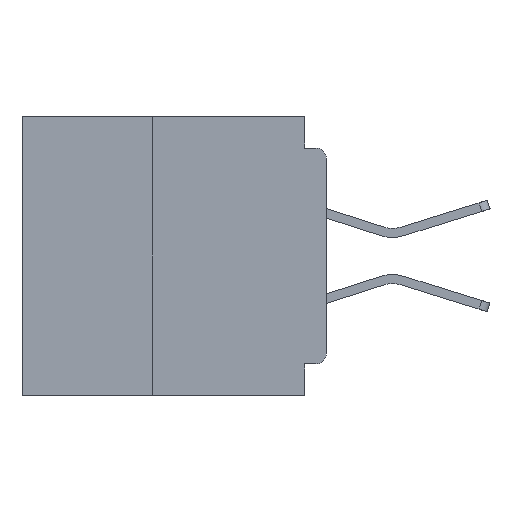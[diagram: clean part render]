
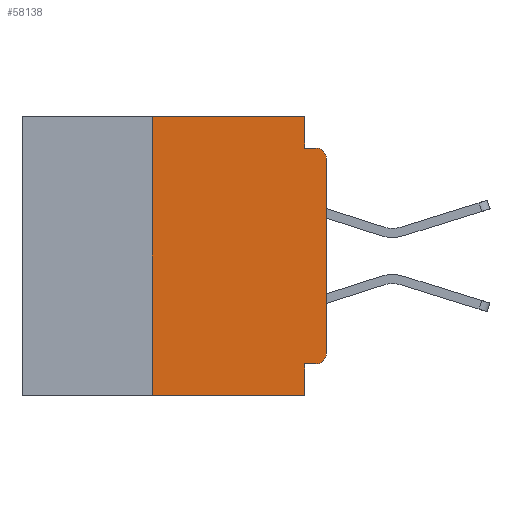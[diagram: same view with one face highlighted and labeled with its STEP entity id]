
A CAD part, left-side view. The second image highlights one B-rep face of the part: STEP entity #58138.
In plain terms, the highlighted planar face has unit normal (-1, 0, 0).
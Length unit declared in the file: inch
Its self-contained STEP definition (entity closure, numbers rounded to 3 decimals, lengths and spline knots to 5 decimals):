
#1489 = CARTESIAN_POINT ( 'NONE',  ( 0., 0., -0.06 ) ) ;
#2275 = CARTESIAN_POINT ( 'NONE',  ( 0., 0.031, 0. ) ) ;
#2731 = ORIENTED_EDGE ( 'NONE', *, *, #26968, .F. ) ;
#3006 = FACE_OUTER_BOUND ( 'NONE', #5489, .T. ) ;
#3171 = CARTESIAN_POINT ( 'NONE',  ( 0., 0.437, -0.4 ) ) ;
#3813 = VERTEX_POINT ( 'NONE', #17978 ) ;
#4957 = DIRECTION ( 'NONE',  ( 0., 0., 1. ) ) ;
#5137 = EDGE_CURVE ( 'NONE', #26062, #48264, #26834, .T. ) ;
#5148 = VECTOR ( 'NONE', #8338, 39.37008 ) ;
#5489 = EDGE_LOOP ( 'NONE', ( #11112, #23788, #39793, #32274, #34479, #48399, #5959, #2731, #17538, #36929 ) ) ;
#5654 = DIRECTION ( 'NONE',  ( 0., -1., 0. ) ) ;
#5959 = ORIENTED_EDGE ( 'NONE', *, *, #33582, .T. ) ;
#6021 = VERTEX_POINT ( 'NONE', #2275 ) ;
#7006 = EDGE_CURVE ( 'NONE', #56599, #48264, #22376, .T. ) ;
#8338 = DIRECTION ( 'NONE',  ( 0., -1., 0. ) ) ;
#9839 = VERTEX_POINT ( 'NONE', #38324 ) ;
#11072 = CARTESIAN_POINT ( 'NONE',  ( 0., 0.015, -0.34 ) ) ;
#11112 = ORIENTED_EDGE ( 'NONE', *, *, #22814, .T. ) ;
#13249 = CARTESIAN_POINT ( 'NONE',  ( 0., 0., -0.34 ) ) ;
#13445 = PLANE ( 'NONE',  #36985 ) ;
#14200 = CARTESIAN_POINT ( 'NONE',  ( 0., 0.015, -0.355 ) ) ;
#14259 = CARTESIAN_POINT ( 'NONE',  ( 0., 0.015, -0.06 ) ) ;
#14499 = LINE ( 'NONE', #41904, #27992 ) ;
#14874 = DIRECTION ( 'NONE',  ( 0., 1., 0. ) ) ;
#15630 = DIRECTION ( 'NONE',  ( 0., 0., -1. ) ) ;
#15674 = VECTOR ( 'NONE', #28658, 39.37008 ) ;
#17348 = CARTESIAN_POINT ( 'NONE',  ( 0., 0.031, -0.355 ) ) ;
#17538 = ORIENTED_EDGE ( 'NONE', *, *, #51040, .F. ) ;
#17776 = EDGE_CURVE ( 'NONE', #9839, #3813, #32644, .T. ) ;
#17978 = CARTESIAN_POINT ( 'NONE',  ( 0., 0.25, 0. ) ) ;
#18858 = DIRECTION ( 'NONE',  ( 0., 0., -1. ) ) ;
#21044 = AXIS2_PLACEMENT_3D ( 'NONE', #11072, #42638, #15630 ) ;
#22376 = LINE ( 'NONE', #41868, #56713 ) ;
#22814 = EDGE_CURVE ( 'NONE', #41666, #26062, #39669, .T. ) ;
#23788 = ORIENTED_EDGE ( 'NONE', *, *, #5137, .T. ) ;
#25948 = VECTOR ( 'NONE', #48443, 39.37008 ) ;
#26062 = VERTEX_POINT ( 'NONE', #1489 ) ;
#26834 = CIRCLE ( 'NONE', #52191, 0.015 ) ;
#26889 = CIRCLE ( 'NONE', #21044, 0.015 ) ;
#26968 = EDGE_CURVE ( 'NONE', #44136, #51955, #39863, .T. ) ;
#27157 = DIRECTION ( 'NONE',  ( 0., 0., -1. ) ) ;
#27673 = CARTESIAN_POINT ( 'NONE',  ( 0., 0.25, -0.4 ) ) ;
#27992 = VECTOR ( 'NONE', #14874, 39.37008 ) ;
#28658 = DIRECTION ( 'NONE',  ( 0., 0., 1. ) ) ;
#29350 = LINE ( 'NONE', #39966, #5148 ) ;
#31251 = VECTOR ( 'NONE', #4957, 39.37008 ) ;
#32274 = ORIENTED_EDGE ( 'NONE', *, *, #48488, .F. ) ;
#32644 = LINE ( 'NONE', #27673, #31251 ) ;
#33582 = EDGE_CURVE ( 'NONE', #9839, #51955, #49735, .T. ) ;
#33800 = CARTESIAN_POINT ( 'NONE',  ( 0., 0.031, -0.045 ) ) ;
#33831 = VERTEX_POINT ( 'NONE', #14200 ) ;
#34479 = ORIENTED_EDGE ( 'NONE', *, *, #52571, .F. ) ;
#35772 = CARTESIAN_POINT ( 'NONE',  ( 0., 0.031, 0. ) ) ;
#36929 = ORIENTED_EDGE ( 'NONE', *, *, #55358, .T. ) ;
#36985 = AXIS2_PLACEMENT_3D ( 'NONE', #58286, #53965, #27157 ) ;
#38324 = CARTESIAN_POINT ( 'NONE',  ( 0., 0.25, -0.4 ) ) ;
#38477 = VECTOR ( 'NONE', #58525, 39.37008 ) ;
#39669 = LINE ( 'NONE', #55275, #15674 ) ;
#39793 = ORIENTED_EDGE ( 'NONE', *, *, #7006, .F. ) ;
#39863 = LINE ( 'NONE', #45038, #38477 ) ;
#39966 = CARTESIAN_POINT ( 'NONE',  ( 0., 0.437, 0. ) ) ;
#40301 = DIRECTION ( 'NONE',  ( 0., 0., -1. ) ) ;
#41666 = VERTEX_POINT ( 'NONE', #13249 ) ;
#41868 = CARTESIAN_POINT ( 'NONE',  ( 0., 0., -0.045 ) ) ;
#41904 = CARTESIAN_POINT ( 'NONE',  ( 0., 0., -0.355 ) ) ;
#42638 = DIRECTION ( 'NONE',  ( -1., 0., 0. ) ) ;
#44136 = VERTEX_POINT ( 'NONE', #17348 ) ;
#45038 = CARTESIAN_POINT ( 'NONE',  ( 0., 0.031, -0.4 ) ) ;
#45787 = DIRECTION ( 'NONE',  ( -1., 0., 0. ) ) ;
#48264 = VERTEX_POINT ( 'NONE', #52040 ) ;
#48399 = ORIENTED_EDGE ( 'NONE', *, *, #17776, .F. ) ;
#48443 = DIRECTION ( 'NONE',  ( 0., -1., 0. ) ) ;
#48488 = EDGE_CURVE ( 'NONE', #6021, #56599, #57629, .T. ) ;
#49735 = LINE ( 'NONE', #3171, #25948 ) ;
#51040 = EDGE_CURVE ( 'NONE', #33831, #44136, #14499, .T. ) ;
#51955 = VERTEX_POINT ( 'NONE', #53712 ) ;
#52040 = CARTESIAN_POINT ( 'NONE',  ( 0., 0.015, -0.045 ) ) ;
#52191 = AXIS2_PLACEMENT_3D ( 'NONE', #14259, #45787, #18858 ) ;
#52571 = EDGE_CURVE ( 'NONE', #3813, #6021, #29350, .T. ) ;
#53712 = CARTESIAN_POINT ( 'NONE',  ( 0., 0.031, -0.4 ) ) ;
#53965 = DIRECTION ( 'NONE',  ( 1., 0., 0. ) ) ;
#55275 = CARTESIAN_POINT ( 'NONE',  ( 0., 0., 0. ) ) ;
#55358 = EDGE_CURVE ( 'NONE', #33831, #41666, #26889, .T. ) ;
#56211 = VECTOR ( 'NONE', #40301, 39.37008 ) ;
#56599 = VERTEX_POINT ( 'NONE', #33800 ) ;
#56713 = VECTOR ( 'NONE', #5654, 39.37008 ) ;
#57629 = LINE ( 'NONE', #35772, #56211 ) ;
#58138 = ADVANCED_FACE ( 'NONE', ( #3006 ), #13445, .F. ) ;
#58286 = CARTESIAN_POINT ( 'NONE',  ( 0., 0.437, 0. ) ) ;
#58525 = DIRECTION ( 'NONE',  ( 0., 0., -1. ) ) ;
